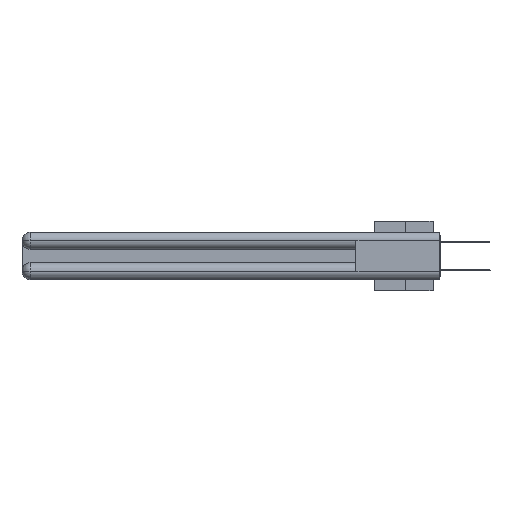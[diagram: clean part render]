
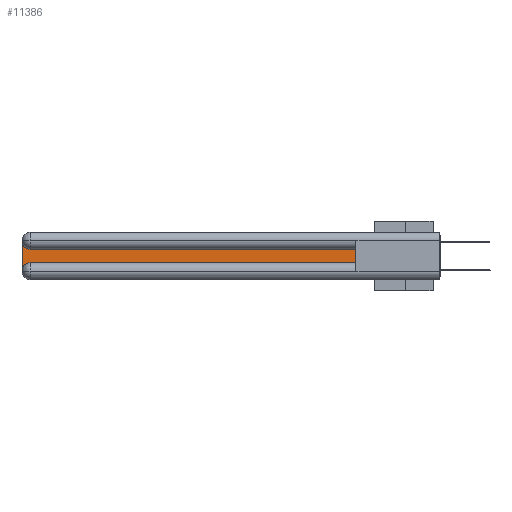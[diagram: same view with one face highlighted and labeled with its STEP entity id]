
A CAD part, left-side view. The second image highlights one B-rep face of the part: STEP entity #11386.
In plain terms, the highlighted planar face has unit normal (-1, 0, 0).
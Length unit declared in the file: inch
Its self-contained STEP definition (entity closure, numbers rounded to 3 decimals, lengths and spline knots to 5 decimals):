
#922 = VECTOR ( 'NONE', #14801, 39.37008 ) ;
#2451 = VERTEX_POINT ( 'NONE', #33218 ) ;
#2536 = CARTESIAN_POINT ( 'NONE',  ( 0.075, 0.6, -0.1225 ) ) ;
#2596 = CARTESIAN_POINT ( 'NONE',  ( 0.075, 2.94, -0.0625 ) ) ;
#2646 = VERTEX_POINT ( 'NONE', #14707 ) ;
#2810 = DIRECTION ( 'NONE',  ( 0., 0., -1. ) ) ;
#3479 = ORIENTED_EDGE ( 'NONE', *, *, #8404, .T. ) ;
#4727 = AXIS2_PLACEMENT_3D ( 'NONE', #25411, #9723, #19216 ) ;
#5109 = EDGE_CURVE ( 'NONE', #29462, #2646, #31686, .T. ) ;
#5554 = VECTOR ( 'NONE', #19122, 39.37008 ) ;
#5864 = FACE_OUTER_BOUND ( 'NONE', #25618, .T. ) ;
#7259 = CARTESIAN_POINT ( 'NONE',  ( 0.075, 0.6, -0.1225 ) ) ;
#7930 = CARTESIAN_POINT ( 'NONE',  ( 0.075, 3., -0.2775 ) ) ;
#8296 = CIRCLE ( 'NONE', #4727, 0.06 ) ;
#8404 = EDGE_CURVE ( 'NONE', #2451, #14483, #26244, .T. ) ;
#9395 = EDGE_CURVE ( 'NONE', #39247, #2451, #18858, .T. ) ;
#9723 = DIRECTION ( 'NONE',  ( 1., 0., 0. ) ) ;
#9996 = ORIENTED_EDGE ( 'NONE', *, *, #18537, .T. ) ;
#11221 = EDGE_CURVE ( 'NONE', #14483, #29462, #34912, .T. ) ;
#11386 = ADVANCED_FACE ( 'NONE', ( #5864 ), #21405, .F. ) ;
#11915 = DIRECTION ( 'NONE',  ( 1., 0., 0. ) ) ;
#11938 = AXIS2_PLACEMENT_3D ( 'NONE', #14813, #11915, #2810 ) ;
#12812 = CARTESIAN_POINT ( 'NONE',  ( 0.075, 0.6, -0.2175 ) ) ;
#13357 = AXIS2_PLACEMENT_3D ( 'NONE', #2596, #18404, #21324 ) ;
#14483 = VERTEX_POINT ( 'NONE', #7259 ) ;
#14557 = CARTESIAN_POINT ( 'NONE',  ( 0.075, 0.6, -0.2175 ) ) ;
#14707 = CARTESIAN_POINT ( 'NONE',  ( 0.075, 3., -0.0625 ) ) ;
#14801 = DIRECTION ( 'NONE',  ( 0., 1., 0. ) ) ;
#14813 = CARTESIAN_POINT ( 'NONE',  ( 0.075, 3., -0.1225 ) ) ;
#16832 = ORIENTED_EDGE ( 'NONE', *, *, #17215, .T. ) ;
#17215 = EDGE_CURVE ( 'NONE', #2646, #17323, #36472, .T. ) ;
#17323 = VERTEX_POINT ( 'NONE', #7930 ) ;
#17925 = VECTOR ( 'NONE', #36512, 39.37008 ) ;
#18404 = DIRECTION ( 'NONE',  ( 1., 0., 0. ) ) ;
#18537 = EDGE_CURVE ( 'NONE', #17323, #39247, #8296, .T. ) ;
#18858 = LINE ( 'NONE', #12812, #5554 ) ;
#19122 = DIRECTION ( 'NONE',  ( 0., -1., 0. ) ) ;
#19216 = DIRECTION ( 'NONE',  ( 0., 0., -1. ) ) ;
#19300 = ORIENTED_EDGE ( 'NONE', *, *, #5109, .T. ) ;
#21324 = DIRECTION ( 'NONE',  ( 0., 0., -1. ) ) ;
#21405 = PLANE ( 'NONE',  #11938 ) ;
#25411 = CARTESIAN_POINT ( 'NONE',  ( 0.075, 2.94, -0.2775 ) ) ;
#25618 = EDGE_LOOP ( 'NONE', ( #31181, #19300, #16832, #9996, #40254, #3479 ) ) ;
#26244 = LINE ( 'NONE', #14557, #17925 ) ;
#26719 = CARTESIAN_POINT ( 'NONE',  ( 0.075, 2.94, -0.1225 ) ) ;
#27015 = CARTESIAN_POINT ( 'NONE',  ( 0.075, 3., -0.2175 ) ) ;
#28121 = VECTOR ( 'NONE', #33312, 39.37008 ) ;
#29462 = VERTEX_POINT ( 'NONE', #26719 ) ;
#31181 = ORIENTED_EDGE ( 'NONE', *, *, #11221, .T. ) ;
#31686 = CIRCLE ( 'NONE', #13357, 0.06 ) ;
#33218 = CARTESIAN_POINT ( 'NONE',  ( 0.075, 0.6, -0.2175 ) ) ;
#33312 = DIRECTION ( 'NONE',  ( 0., 0., -1. ) ) ;
#34912 = LINE ( 'NONE', #2536, #922 ) ;
#35989 = CARTESIAN_POINT ( 'NONE',  ( 0.075, 2.94, -0.2175 ) ) ;
#36472 = LINE ( 'NONE', #27015, #28121 ) ;
#36512 = DIRECTION ( 'NONE',  ( 0., 0., 1. ) ) ;
#39247 = VERTEX_POINT ( 'NONE', #35989 ) ;
#40254 = ORIENTED_EDGE ( 'NONE', *, *, #9395, .T. ) ;
